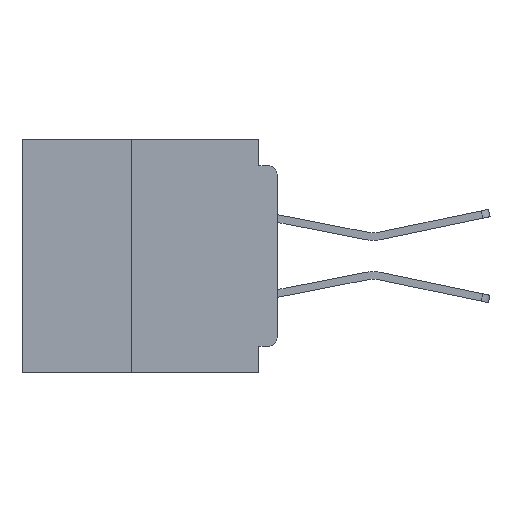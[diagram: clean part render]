
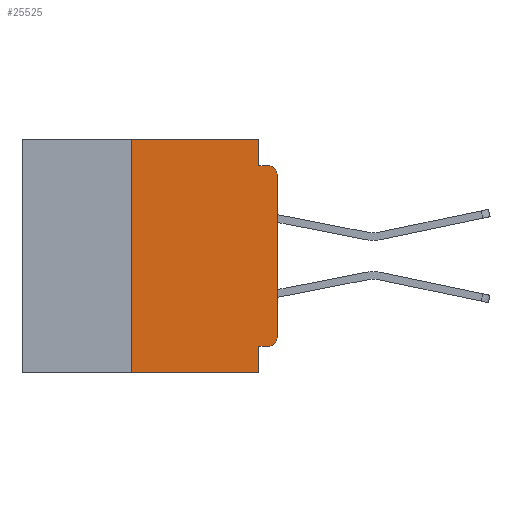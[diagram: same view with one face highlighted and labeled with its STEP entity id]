
A CAD part, left-side view. The second image highlights one B-rep face of the part: STEP entity #25525.
In plain terms, the highlighted planar face has unit normal (-1, 0, 0).
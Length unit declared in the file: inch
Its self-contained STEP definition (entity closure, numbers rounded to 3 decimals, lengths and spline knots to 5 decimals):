
#348 = CARTESIAN_POINT ( 'NONE',  ( 0., 0.437, 0. ) ) ;
#868 = DIRECTION ( 'NONE',  ( 0., 0., -1. ) ) ;
#883 = DIRECTION ( 'NONE',  ( 0., 0., 1. ) ) ;
#1875 = EDGE_CURVE ( 'NONE', #39752, #16581, #37995, .T. ) ;
#2460 = CARTESIAN_POINT ( 'NONE',  ( 0., 0.031, -0.4 ) ) ;
#2728 = LINE ( 'NONE', #42530, #11752 ) ;
#4205 = DIRECTION ( 'NONE',  ( 1., 0., 0. ) ) ;
#4294 = FACE_OUTER_BOUND ( 'NONE', #19479, .T. ) ;
#4974 = VECTOR ( 'NONE', #20101, 39.37008 ) ;
#6038 = LINE ( 'NONE', #26826, #4974 ) ;
#6049 = CARTESIAN_POINT ( 'NONE',  ( 0., 0.031, 0. ) ) ;
#6159 = AXIS2_PLACEMENT_3D ( 'NONE', #41072, #21161, #868 ) ;
#6418 = DIRECTION ( 'NONE',  ( 0., 0., -1. ) ) ;
#8513 = ORIENTED_EDGE ( 'NONE', *, *, #33587, .T. ) ;
#8914 = DIRECTION ( 'NONE',  ( 0., 0., 1. ) ) ;
#9040 = CARTESIAN_POINT ( 'NONE',  ( 0., 0.25, -0.4 ) ) ;
#9069 = ORIENTED_EDGE ( 'NONE', *, *, #32083, .F. ) ;
#9110 = CARTESIAN_POINT ( 'NONE',  ( 0., 0.031, -0.355 ) ) ;
#9149 = LINE ( 'NONE', #29046, #18096 ) ;
#9769 = CIRCLE ( 'NONE', #31070, 0.015 ) ;
#10750 = CARTESIAN_POINT ( 'NONE',  ( 0., 0.015, -0.355 ) ) ;
#11199 = ORIENTED_EDGE ( 'NONE', *, *, #20879, .F. ) ;
#11311 = VECTOR ( 'NONE', #6418, 39.37008 ) ;
#11752 = VECTOR ( 'NONE', #33520, 39.37008 ) ;
#12823 = CARTESIAN_POINT ( 'NONE',  ( 0., 0.015, -0.045 ) ) ;
#13320 = CARTESIAN_POINT ( 'NONE',  ( 0., 0.031, -0.045 ) ) ;
#13763 = ORIENTED_EDGE ( 'NONE', *, *, #41882, .F. ) ;
#15558 = VERTEX_POINT ( 'NONE', #2460 ) ;
#16581 = VERTEX_POINT ( 'NONE', #13320 ) ;
#18024 = ORIENTED_EDGE ( 'NONE', *, *, #29856, .T. ) ;
#18039 = VERTEX_POINT ( 'NONE', #10750 ) ;
#18096 = VECTOR ( 'NONE', #8914, 39.37008 ) ;
#18444 = LINE ( 'NONE', #39922, #26326 ) ;
#18643 = DIRECTION ( 'NONE',  ( -1., 0., 0. ) ) ;
#19197 = CARTESIAN_POINT ( 'NONE',  ( 0., 0.25, 0. ) ) ;
#19334 = EDGE_CURVE ( 'NONE', #43402, #39752, #22457, .T. ) ;
#19479 = EDGE_LOOP ( 'NONE', ( #8513, #37337, #13763, #31639, #23800, #9069, #18024, #11199, #37881, #21209 ) ) ;
#20101 = DIRECTION ( 'NONE',  ( 0., -1., 0. ) ) ;
#20650 = DIRECTION ( 'NONE',  ( 0., -1., 0. ) ) ;
#20812 = VERTEX_POINT ( 'NONE', #9040 ) ;
#20879 = EDGE_CURVE ( 'NONE', #22022, #15558, #2728, .T. ) ;
#21161 = DIRECTION ( 'NONE',  ( -1., 0., 0. ) ) ;
#21209 = ORIENTED_EDGE ( 'NONE', *, *, #41569, .T. ) ;
#21571 = CIRCLE ( 'NONE', #6159, 0.015 ) ;
#22022 = VERTEX_POINT ( 'NONE', #9110 ) ;
#22189 = AXIS2_PLACEMENT_3D ( 'NONE', #34467, #4205, #41109 ) ;
#22457 = LINE ( 'NONE', #348, #38067 ) ;
#23800 = ORIENTED_EDGE ( 'NONE', *, *, #19334, .F. ) ;
#25333 = VECTOR ( 'NONE', #883, 39.37008 ) ;
#25525 = ADVANCED_FACE ( 'NONE', ( #4294 ), #37796, .F. ) ;
#26326 = VECTOR ( 'NONE', #29943, 39.37008 ) ;
#26826 = CARTESIAN_POINT ( 'NONE',  ( 0., 0., -0.045 ) ) ;
#27039 = VERTEX_POINT ( 'NONE', #12823 ) ;
#27220 = LINE ( 'NONE', #36960, #42754 ) ;
#27653 = VERTEX_POINT ( 'NONE', #42914 ) ;
#28836 = EDGE_CURVE ( 'NONE', #27653, #27039, #21571, .T. ) ;
#29046 = CARTESIAN_POINT ( 'NONE',  ( 0., 0.25, -0.4 ) ) ;
#29385 = VERTEX_POINT ( 'NONE', #34398 ) ;
#29856 = EDGE_CURVE ( 'NONE', #20812, #15558, #27220, .T. ) ;
#29943 = DIRECTION ( 'NONE',  ( 0., 1., 0. ) ) ;
#31070 = AXIS2_PLACEMENT_3D ( 'NONE', #38619, #18643, #41929 ) ;
#31105 = CARTESIAN_POINT ( 'NONE',  ( 0., 0., 0. ) ) ;
#31639 = ORIENTED_EDGE ( 'NONE', *, *, #1875, .F. ) ;
#32083 = EDGE_CURVE ( 'NONE', #20812, #43402, #9149, .T. ) ;
#33520 = DIRECTION ( 'NONE',  ( 0., 0., -1. ) ) ;
#33587 = EDGE_CURVE ( 'NONE', #29385, #27653, #34170, .T. ) ;
#34170 = LINE ( 'NONE', #31105, #25333 ) ;
#34398 = CARTESIAN_POINT ( 'NONE',  ( 0., 0., -0.34 ) ) ;
#34467 = CARTESIAN_POINT ( 'NONE',  ( 0., 0.437, 0. ) ) ;
#34691 = EDGE_CURVE ( 'NONE', #18039, #22022, #18444, .T. ) ;
#36960 = CARTESIAN_POINT ( 'NONE',  ( 0., 0.437, -0.4 ) ) ;
#37102 = DIRECTION ( 'NONE',  ( 0., -1., 0. ) ) ;
#37337 = ORIENTED_EDGE ( 'NONE', *, *, #28836, .T. ) ;
#37796 = PLANE ( 'NONE',  #22189 ) ;
#37881 = ORIENTED_EDGE ( 'NONE', *, *, #34691, .F. ) ;
#37995 = LINE ( 'NONE', #6049, #11311 ) ;
#38067 = VECTOR ( 'NONE', #20650, 39.37008 ) ;
#38619 = CARTESIAN_POINT ( 'NONE',  ( 0., 0.015, -0.34 ) ) ;
#39752 = VERTEX_POINT ( 'NONE', #41783 ) ;
#39922 = CARTESIAN_POINT ( 'NONE',  ( 0., 0., -0.355 ) ) ;
#41072 = CARTESIAN_POINT ( 'NONE',  ( 0., 0.015, -0.06 ) ) ;
#41109 = DIRECTION ( 'NONE',  ( 0., 0., -1. ) ) ;
#41569 = EDGE_CURVE ( 'NONE', #18039, #29385, #9769, .T. ) ;
#41783 = CARTESIAN_POINT ( 'NONE',  ( 0., 0.031, 0. ) ) ;
#41882 = EDGE_CURVE ( 'NONE', #16581, #27039, #6038, .T. ) ;
#41929 = DIRECTION ( 'NONE',  ( 0., 0., -1. ) ) ;
#42530 = CARTESIAN_POINT ( 'NONE',  ( 0., 0.031, -0.4 ) ) ;
#42754 = VECTOR ( 'NONE', #37102, 39.37008 ) ;
#42914 = CARTESIAN_POINT ( 'NONE',  ( 0., 0., -0.06 ) ) ;
#43402 = VERTEX_POINT ( 'NONE', #19197 ) ;
